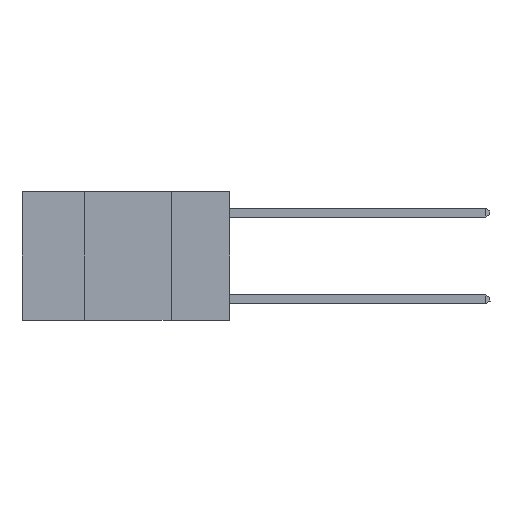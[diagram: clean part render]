
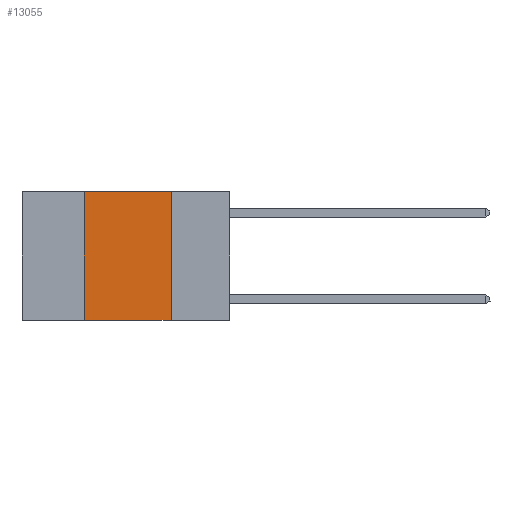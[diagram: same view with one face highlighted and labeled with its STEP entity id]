
A CAD part, left-side view. The second image highlights one B-rep face of the part: STEP entity #13055.
In plain terms, the highlighted planar face has unit normal (-1, 0, 0).
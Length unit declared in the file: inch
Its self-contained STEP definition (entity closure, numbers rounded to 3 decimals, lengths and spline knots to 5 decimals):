
#147 = LINE ( 'NONE', #12955, #7389 ) ;
#857 = PLANE ( 'NONE',  #14896 ) ;
#977 = DIRECTION ( 'NONE',  ( 0., -1., 0. ) ) ;
#1209 = VERTEX_POINT ( 'NONE', #15344 ) ;
#1811 = DIRECTION ( 'NONE',  ( 0., 0., -1. ) ) ;
#2574 = VERTEX_POINT ( 'NONE', #17883 ) ;
#2863 = VECTOR ( 'NONE', #19518, 39.37008 ) ;
#3109 = CARTESIAN_POINT ( 'NONE',  ( 0., 0.42, -0.37 ) ) ;
#3881 = CARTESIAN_POINT ( 'NONE',  ( 0., 0.6, 0. ) ) ;
#4927 = ORIENTED_EDGE ( 'NONE', *, *, #13743, .F. ) ;
#5404 = EDGE_CURVE ( 'NONE', #14022, #2574, #147, .T. ) ;
#5517 = DIRECTION ( 'NONE',  ( 1., 0., 0. ) ) ;
#5560 = CARTESIAN_POINT ( 'NONE',  ( 0., 0.6, 0. ) ) ;
#5767 = CARTESIAN_POINT ( 'NONE',  ( 0., 0.6, -0.37 ) ) ;
#6407 = LINE ( 'NONE', #9544, #14089 ) ;
#7389 = VECTOR ( 'NONE', #11366, 39.37008 ) ;
#9544 = CARTESIAN_POINT ( 'NONE',  ( 0., 0.17, 0. ) ) ;
#10239 = EDGE_CURVE ( 'NONE', #1209, #15416, #6407, .T. ) ;
#10666 = CARTESIAN_POINT ( 'NONE',  ( 0., 0.17, -0.37 ) ) ;
#11366 = DIRECTION ( 'NONE',  ( 0., 0., 1. ) ) ;
#11600 = LINE ( 'NONE', #5767, #2863 ) ;
#12955 = CARTESIAN_POINT ( 'NONE',  ( 0., 0.42, 0. ) ) ;
#13042 = FACE_OUTER_BOUND ( 'NONE', #16928, .T. ) ;
#13055 = ADVANCED_FACE ( 'NONE', ( #13042 ), #857, .F. ) ;
#13145 = ORIENTED_EDGE ( 'NONE', *, *, #5404, .F. ) ;
#13743 = EDGE_CURVE ( 'NONE', #2574, #1209, #16809, .T. ) ;
#14022 = VERTEX_POINT ( 'NONE', #3109 ) ;
#14089 = VECTOR ( 'NONE', #1811, 39.37008 ) ;
#14896 = AXIS2_PLACEMENT_3D ( 'NONE', #3881, #5517, #16242 ) ;
#15344 = CARTESIAN_POINT ( 'NONE',  ( 0., 0.17, 0. ) ) ;
#15416 = VERTEX_POINT ( 'NONE', #10666 ) ;
#16242 = DIRECTION ( 'NONE',  ( 0., 0., -1. ) ) ;
#16321 = VECTOR ( 'NONE', #977, 39.37008 ) ;
#16697 = ORIENTED_EDGE ( 'NONE', *, *, #10239, .F. ) ;
#16710 = EDGE_CURVE ( 'NONE', #14022, #15416, #11600, .T. ) ;
#16809 = LINE ( 'NONE', #5560, #16321 ) ;
#16928 = EDGE_LOOP ( 'NONE', ( #16697, #4927, #13145, #18122 ) ) ;
#17883 = CARTESIAN_POINT ( 'NONE',  ( 0., 0.42, 0. ) ) ;
#18122 = ORIENTED_EDGE ( 'NONE', *, *, #16710, .T. ) ;
#19518 = DIRECTION ( 'NONE',  ( 0., -1., 0. ) ) ;
